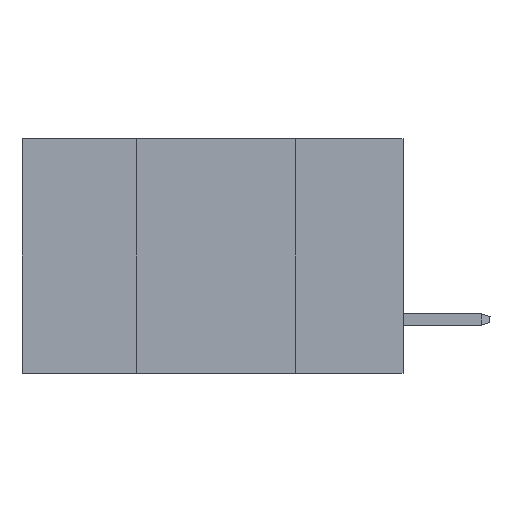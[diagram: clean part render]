
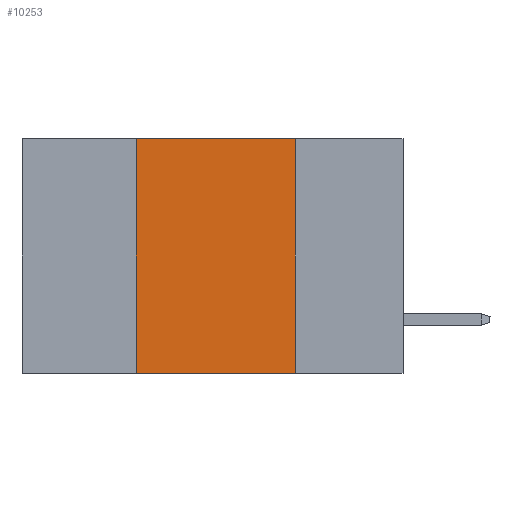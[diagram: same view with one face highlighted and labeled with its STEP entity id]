
A CAD part, left-side view. The second image highlights one B-rep face of the part: STEP entity #10253.
In plain terms, the highlighted planar face has unit normal (-1, 0, 0).
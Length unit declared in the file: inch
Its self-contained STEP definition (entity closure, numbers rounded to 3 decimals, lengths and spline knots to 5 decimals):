
#826 = ORIENTED_EDGE ( 'NONE', *, *, #9414, .T. ) ;
#1566 = VECTOR ( 'NONE', #38976, 39.37008 ) ;
#3824 = DIRECTION ( 'NONE',  ( 0., -1., 0. ) ) ;
#4656 = VECTOR ( 'NONE', #3824, 39.37008 ) ;
#5106 = VERTEX_POINT ( 'NONE', #19498 ) ;
#5500 = DIRECTION ( 'NONE',  ( 0., -1., 0. ) ) ;
#8379 = ORIENTED_EDGE ( 'NONE', *, *, #9484, .F. ) ;
#8908 = LINE ( 'NONE', #15970, #37522 ) ;
#9414 = EDGE_CURVE ( 'NONE', #25994, #11908, #36379, .T. ) ;
#9484 = EDGE_CURVE ( 'NONE', #25994, #12048, #8908, .T. ) ;
#9641 = LINE ( 'NONE', #35742, #1566 ) ;
#10253 = ADVANCED_FACE ( 'NONE', ( #21639 ), #21223, .F. ) ;
#11477 = AXIS2_PLACEMENT_3D ( 'NONE', #34700, #37922, #37712 ) ;
#11908 = VERTEX_POINT ( 'NONE', #30374 ) ;
#11977 = CARTESIAN_POINT ( 'NONE',  ( 0., 0.42, 0. ) ) ;
#12048 = VERTEX_POINT ( 'NONE', #11977 ) ;
#12560 = EDGE_CURVE ( 'NONE', #12048, #5106, #21760, .T. ) ;
#15970 = CARTESIAN_POINT ( 'NONE',  ( 0., 0.42, 0. ) ) ;
#17874 = EDGE_CURVE ( 'NONE', #5106, #11908, #9641, .T. ) ;
#19498 = CARTESIAN_POINT ( 'NONE',  ( 0., 0.17, 0. ) ) ;
#20100 = CARTESIAN_POINT ( 'NONE',  ( 0., 0.6, -0.37 ) ) ;
#21223 = PLANE ( 'NONE',  #11477 ) ;
#21639 = FACE_OUTER_BOUND ( 'NONE', #35479, .T. ) ;
#21760 = LINE ( 'NONE', #34823, #36890 ) ;
#23006 = ORIENTED_EDGE ( 'NONE', *, *, #17874, .F. ) ;
#25994 = VERTEX_POINT ( 'NONE', #38713 ) ;
#30374 = CARTESIAN_POINT ( 'NONE',  ( 0., 0.17, -0.37 ) ) ;
#34700 = CARTESIAN_POINT ( 'NONE',  ( 0., 0.6, 0. ) ) ;
#34823 = CARTESIAN_POINT ( 'NONE',  ( 0., 0.6, 0. ) ) ;
#35479 = EDGE_LOOP ( 'NONE', ( #23006, #36610, #8379, #826 ) ) ;
#35742 = CARTESIAN_POINT ( 'NONE',  ( 0., 0.17, 0. ) ) ;
#36379 = LINE ( 'NONE', #20100, #4656 ) ;
#36610 = ORIENTED_EDGE ( 'NONE', *, *, #12560, .F. ) ;
#36890 = VECTOR ( 'NONE', #5500, 39.37008 ) ;
#37522 = VECTOR ( 'NONE', #38656, 39.37008 ) ;
#37712 = DIRECTION ( 'NONE',  ( 0., 0., -1. ) ) ;
#37922 = DIRECTION ( 'NONE',  ( 1., 0., 0. ) ) ;
#38656 = DIRECTION ( 'NONE',  ( 0., 0., 1. ) ) ;
#38713 = CARTESIAN_POINT ( 'NONE',  ( 0., 0.42, -0.37 ) ) ;
#38976 = DIRECTION ( 'NONE',  ( 0., 0., -1. ) ) ;
